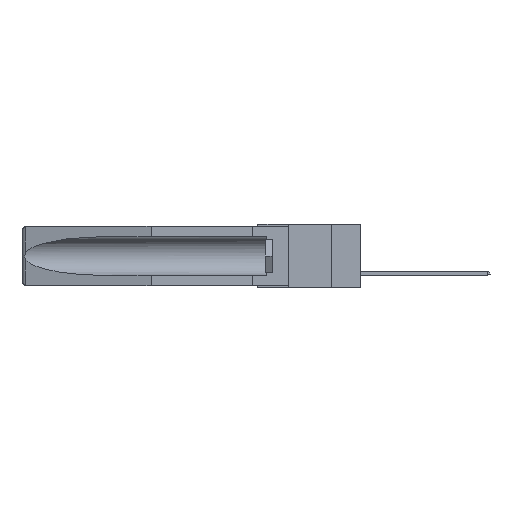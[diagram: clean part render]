
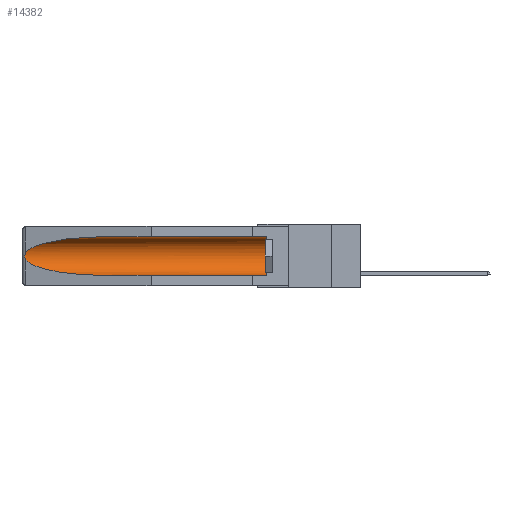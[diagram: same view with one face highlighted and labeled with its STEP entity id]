
A CAD part, left-side view. The second image highlights one B-rep face of the part: STEP entity #14382.
In plain terms, the highlighted cylindrical face has radius 2.857 mm (diameter 5.715 mm), a partial arc.
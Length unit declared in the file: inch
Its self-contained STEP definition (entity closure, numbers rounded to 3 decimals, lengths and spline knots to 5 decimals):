
#530 = EDGE_CURVE ( 'NONE', #13484, #634, #16569, .T. ) ;
#634 = VERTEX_POINT ( 'NONE', #1528 ) ;
#886 = ORIENTED_EDGE ( 'NONE', *, *, #22837, .T. ) ;
#1528 = CARTESIAN_POINT ( 'NONE',  ( 0.155, 0.126, -0.059 ) ) ;
#1646 = CARTESIAN_POINT ( 'NONE',  ( 0.155, 0.126, -0.284 ) ) ;
#1755 = DIRECTION ( 'NONE',  ( 0., 0., 1. ) ) ;
#4060 = CARTESIAN_POINT ( 'NONE',  ( 0.2673, 1.5327, -0.16383 ) ) ;
#4145 = ORIENTED_EDGE ( 'NONE', *, *, #23339, .T. ) ;
#4235 = CARTESIAN_POINT ( 'NONE',  ( 0.26537, 1.52718, -0.19328 ) ) ;
#4833 = CARTESIAN_POINT ( 'NONE',  ( 0.26537, 1.52718, -0.14972 ) ) ;
#4914 = ORIENTED_EDGE ( 'NONE', *, *, #530, .T. ) ;
#5091 = DIRECTION ( 'NONE',  ( 0., 1., 0. ) ) ;
#5129 = FACE_OUTER_BOUND ( 'NONE', #5395, .T. ) ;
#5395 = EDGE_LOOP ( 'NONE', ( #11708, #886, #4145, #6149, #4914, #11100 ) ) ;
#5485 = CARTESIAN_POINT ( 'NONE',  ( 0.155, 1.07973, -0.284 ) ) ;
#5760 = EDGE_CURVE ( 'NONE', #21981, #15614, #12035, .T. ) ;
#6149 = ORIENTED_EDGE ( 'NONE', *, *, #11717, .F. ) ;
#7021 = DIRECTION ( 'NONE',  ( 0., 1., 0. ) ) ;
#7378 = CARTESIAN_POINT ( 'NONE',  ( 0.26537, 1.52718, -0.19328 ) ) ;
#7864 = CARTESIAN_POINT ( 'NONE',  ( 0.26597, 1.52961, -0.15275 ) ) ;
#7948 = CARTESIAN_POINT ( 'NONE',  ( 0.26537, 1.52718, -0.14972 ) ) ;
#8550 = CARTESIAN_POINT ( 'NONE',  ( 0.25451, 1.48313, -0.09465 ) ) ;
#9180 = CARTESIAN_POINT ( 'NONE',  ( 0.155, -0.30754, -0.059 ) ) ;
#9307 = B_SPLINE_CURVE_WITH_KNOTS ( 'NONE', 3,
 ( #7948, #7864, #13386, #4060, #20798, #19015, #15253, #17257, #9854, #4235 ),
 .UNSPECIFIED., .F., .F.,
 ( 4, 2, 2, 2, 4 ),
 ( 0., 0.00029, 0.00058, 0.00087, 0.00117 ),
 .UNSPECIFIED. ) ;
#9466 = VERTEX_POINT ( 'NONE', #21608 ) ;
#9854 = CARTESIAN_POINT ( 'NONE',  ( 0.26597, 1.5296, -0.19026 ) ) ;
#10456 = DIRECTION ( 'NONE',  ( 0., 0., 1. ) ) ;
#11008 = AXIS2_PLACEMENT_3D ( 'NONE', #18318, #14706, #1755 ) ;
#11100 = ORIENTED_EDGE ( 'NONE', *, *, #17174, .T. ) ;
#11449 = VECTOR ( 'NONE', #7021, 39.37008 ) ;
#11708 = ORIENTED_EDGE ( 'NONE', *, *, #5760, .T. ) ;
#11717 = EDGE_CURVE ( 'NONE', #13484, #9466, #14252, .T. ) ;
#12035 =( BOUNDED_CURVE ( )  B_SPLINE_CURVE ( 3, ( #19455, #21299, #8550, #4833 ),
 .UNSPECIFIED., .F., .F. ) 
 B_SPLINE_CURVE_WITH_KNOTS ( ( 4, 4 ),
 ( 4.71239, 6.08839 ),
 .UNSPECIFIED. ) 
 CURVE ( )  GEOMETRIC_REPRESENTATION_ITEM ( )  RATIONAL_B_SPLINE_CURVE ( ( 1., 0.848, 0.848, 1. ) ) 
 REPRESENTATION_ITEM ( '' )  );
#12775 = CARTESIAN_POINT ( 'NONE',  ( 0.26537, 1.52718, -0.19328 ) ) ;
#13386 = CARTESIAN_POINT ( 'NONE',  ( 0.26654, 1.53092, -0.15636 ) ) ;
#13484 = VERTEX_POINT ( 'NONE', #1646 ) ;
#14252 = LINE ( 'NONE', #22480, #15133 ) ;
#14382 = ADVANCED_FACE ( 'NONE', ( #5129 ), #17467, .F. ) ;
#14653 = CARTESIAN_POINT ( 'NONE',  ( 0.21114, 1.30732, -0.284 ) ) ;
#14706 = DIRECTION ( 'NONE',  ( 0., -1., 0. ) ) ;
#15133 = VECTOR ( 'NONE', #20724, 39.37008 ) ;
#15253 = CARTESIAN_POINT ( 'NONE',  ( 0.2673, 1.53269, -0.17917 ) ) ;
#15283 = CARTESIAN_POINT ( 'NONE',  ( 0.26537, 1.52718, -0.14972 ) ) ;
#15614 = VERTEX_POINT ( 'NONE', #15283 ) ;
#16569 = CIRCLE ( 'NONE', #11008, 0.1125 ) ;
#17087 = AXIS2_PLACEMENT_3D ( 'NONE', #21394, #5091, #10456 ) ;
#17174 = EDGE_CURVE ( 'NONE', #634, #21981, #20087, .T. ) ;
#17257 = CARTESIAN_POINT ( 'NONE',  ( 0.26655, 1.53094, -0.18657 ) ) ;
#17467 = CYLINDRICAL_SURFACE ( 'NONE', #17087, 0.1125 ) ;
#18238 = VERTEX_POINT ( 'NONE', #7378 ) ;
#18318 = CARTESIAN_POINT ( 'NONE',  ( 0.155, 0.126, -0.1715 ) ) ;
#18563 =( BOUNDED_CURVE ( )  B_SPLINE_CURVE ( 3, ( #12775, #23692, #14653, #5485 ),
 .UNSPECIFIED., .F., .F. ) 
 B_SPLINE_CURVE_WITH_KNOTS ( ( 4, 4 ),
 ( 0.1948, 1.5708 ),
 .UNSPECIFIED. ) 
 CURVE ( )  GEOMETRIC_REPRESENTATION_ITEM ( )  RATIONAL_B_SPLINE_CURVE ( ( 1., 0.848, 0.848, 1. ) ) 
 REPRESENTATION_ITEM ( '' )  );
#19015 = CARTESIAN_POINT ( 'NONE',  ( 0.2675, 1.53308, -0.17534 ) ) ;
#19455 = CARTESIAN_POINT ( 'NONE',  ( 0.155, 1.07973, -0.059 ) ) ;
#20087 = LINE ( 'NONE', #9180, #11449 ) ;
#20724 = DIRECTION ( 'NONE',  ( 0., 1., 0. ) ) ;
#20798 = CARTESIAN_POINT ( 'NONE',  ( 0.2675, 1.53308, -0.16763 ) ) ;
#21299 = CARTESIAN_POINT ( 'NONE',  ( 0.21114, 1.30732, -0.059 ) ) ;
#21394 = CARTESIAN_POINT ( 'NONE',  ( 0.155, -0.30754, -0.1715 ) ) ;
#21608 = CARTESIAN_POINT ( 'NONE',  ( 0.155, 1.07973, -0.284 ) ) ;
#21879 = CARTESIAN_POINT ( 'NONE',  ( 0.155, 1.07973, -0.059 ) ) ;
#21981 = VERTEX_POINT ( 'NONE', #21879 ) ;
#22480 = CARTESIAN_POINT ( 'NONE',  ( 0.155, -0.30754, -0.284 ) ) ;
#22837 = EDGE_CURVE ( 'NONE', #15614, #18238, #9307, .T. ) ;
#23339 = EDGE_CURVE ( 'NONE', #18238, #9466, #18563, .T. ) ;
#23692 = CARTESIAN_POINT ( 'NONE',  ( 0.25451, 1.48313, -0.24835 ) ) ;
